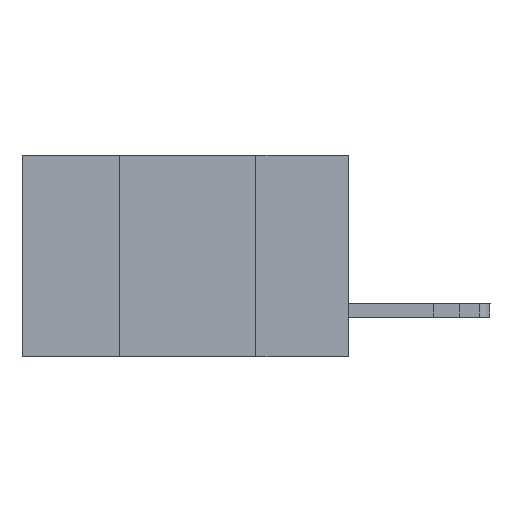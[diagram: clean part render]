
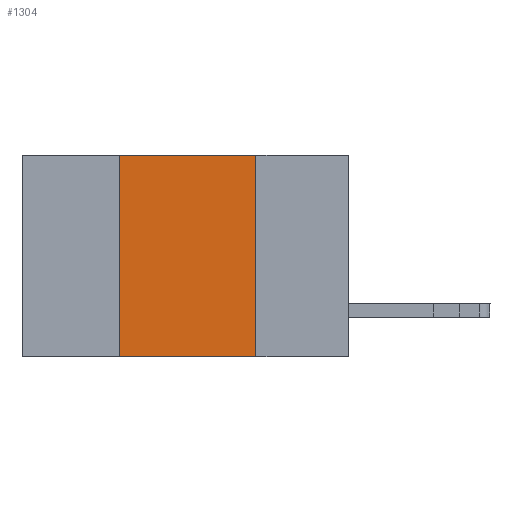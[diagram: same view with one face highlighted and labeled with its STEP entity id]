
A CAD part, left-side view. The second image highlights one B-rep face of the part: STEP entity #1304.
In plain terms, the highlighted planar face has unit normal (-1, 0, 0).
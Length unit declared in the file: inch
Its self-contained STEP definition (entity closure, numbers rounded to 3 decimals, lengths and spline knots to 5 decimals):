
#127 = VERTEX_POINT ( 'NONE', #9889 ) ;
#305 = LINE ( 'NONE', #18179, #3591 ) ;
#438 = VECTOR ( 'NONE', #5564, 39.37008 ) ;
#780 = ORIENTED_EDGE ( 'NONE', *, *, #10444, .F. ) ;
#1304 = ADVANCED_FACE ( 'NONE', ( #20723 ), #6611, .F. ) ;
#3591 = VECTOR ( 'NONE', #9292, 39.37008 ) ;
#4383 = DIRECTION ( 'NONE',  ( 1., 0., 0. ) ) ;
#5564 = DIRECTION ( 'NONE',  ( 0., -1., 0. ) ) ;
#6611 = PLANE ( 'NONE',  #17788 ) ;
#7019 = ORIENTED_EDGE ( 'NONE', *, *, #13221, .T. ) ;
#7983 = CARTESIAN_POINT ( 'NONE',  ( 0., 0.17, -0.37 ) ) ;
#8312 = CARTESIAN_POINT ( 'NONE',  ( 0., 0.42, -0.37 ) ) ;
#8451 = VECTOR ( 'NONE', #18487, 39.37008 ) ;
#9292 = DIRECTION ( 'NONE',  ( 0., -1., 0. ) ) ;
#9488 = LINE ( 'NONE', #7983, #8451 ) ;
#9834 = CARTESIAN_POINT ( 'NONE',  ( 0., 0.42, -0.37 ) ) ;
#9889 = CARTESIAN_POINT ( 'NONE',  ( 0., 0.17, 0. ) ) ;
#10421 = DIRECTION ( 'NONE',  ( 0., 0., 1. ) ) ;
#10444 = EDGE_CURVE ( 'NONE', #21807, #22842, #15339, .T. ) ;
#11012 = CARTESIAN_POINT ( 'NONE',  ( 0., 0.42, 0. ) ) ;
#11251 = VECTOR ( 'NONE', #10421, 39.37008 ) ;
#11583 = VERTEX_POINT ( 'NONE', #19531 ) ;
#11860 = DIRECTION ( 'NONE',  ( 0., 0., -1. ) ) ;
#12341 = LINE ( 'NONE', #16193, #438 ) ;
#13221 = EDGE_CURVE ( 'NONE', #21807, #11583, #12341, .T. ) ;
#13380 = CARTESIAN_POINT ( 'NONE',  ( 0., 0.6, 0. ) ) ;
#15339 = LINE ( 'NONE', #8312, #11251 ) ;
#16193 = CARTESIAN_POINT ( 'NONE',  ( 0., 0.6, -0.37 ) ) ;
#17788 = AXIS2_PLACEMENT_3D ( 'NONE', #13380, #4383, #11860 ) ;
#18179 = CARTESIAN_POINT ( 'NONE',  ( 0., 0.6, 0. ) ) ;
#18266 = ORIENTED_EDGE ( 'NONE', *, *, #20649, .F. ) ;
#18487 = DIRECTION ( 'NONE',  ( 0., 0., -1. ) ) ;
#19531 = CARTESIAN_POINT ( 'NONE',  ( 0., 0.17, -0.37 ) ) ;
#20056 = EDGE_CURVE ( 'NONE', #22842, #127, #305, .T. ) ;
#20649 = EDGE_CURVE ( 'NONE', #127, #11583, #9488, .T. ) ;
#20723 = FACE_OUTER_BOUND ( 'NONE', #22827, .T. ) ;
#20852 = ORIENTED_EDGE ( 'NONE', *, *, #20056, .F. ) ;
#21807 = VERTEX_POINT ( 'NONE', #9834 ) ;
#22827 = EDGE_LOOP ( 'NONE', ( #18266, #20852, #780, #7019 ) ) ;
#22842 = VERTEX_POINT ( 'NONE', #11012 ) ;
